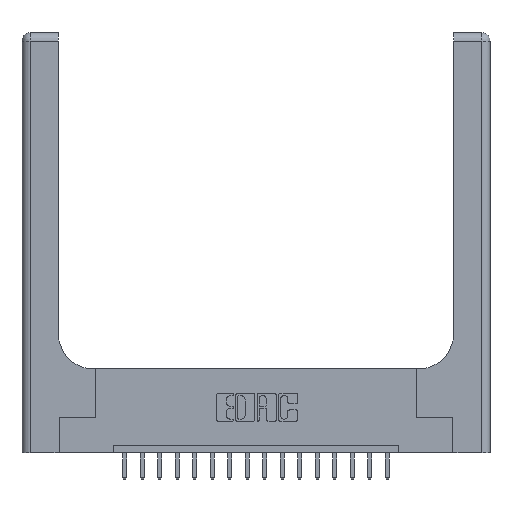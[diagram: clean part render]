
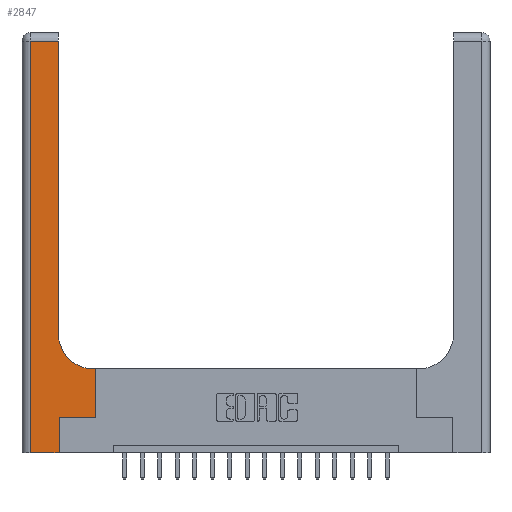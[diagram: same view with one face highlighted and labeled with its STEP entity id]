
A CAD part, top view. The second image highlights one B-rep face of the part: STEP entity #2847.
In plain terms, the highlighted planar face has unit normal (0, 0, 1).
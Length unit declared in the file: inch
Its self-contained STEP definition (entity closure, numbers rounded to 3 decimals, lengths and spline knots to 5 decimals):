
#92 = EDGE_CURVE ( 'NONE', #11981, #3421, #6889, .T. ) ;
#322 = EDGE_LOOP ( 'NONE', ( #5692, #11953, #2452, #6308, #9008, #10097, #18201, #10493, #4284 ) ) ;
#1026 = VERTEX_POINT ( 'NONE', #11431 ) ;
#1510 = DIRECTION ( 'NONE',  ( -1., 0., 0. ) ) ;
#1514 = DIRECTION ( 'NONE',  ( 0., -1., 0. ) ) ;
#1616 = CARTESIAN_POINT ( 'NONE',  ( 0.265, 0., 0.37 ) ) ;
#1628 = VECTOR ( 'NONE', #1514, 39.37008 ) ;
#1690 = CARTESIAN_POINT ( 'NONE',  ( 0., 0., 0.37 ) ) ;
#1723 = LINE ( 'NONE', #10750, #18697 ) ;
#1768 = EDGE_CURVE ( 'NONE', #16068, #11981, #5898, .T. ) ;
#2219 = AXIS2_PLACEMENT_3D ( 'NONE', #16606, #16136, #1510 ) ;
#2291 = VECTOR ( 'NONE', #14707, 39.37008 ) ;
#2452 = ORIENTED_EDGE ( 'NONE', *, *, #1768, .T. ) ;
#2787 = EDGE_CURVE ( 'NONE', #1026, #17145, #7936, .T. ) ;
#2847 = ADVANCED_FACE ( 'NONE', ( #5882 ), #9473, .F. ) ;
#3150 = CARTESIAN_POINT ( 'NONE',  ( 0.06, 2.94, 0.37 ) ) ;
#3396 = CARTESIAN_POINT ( 'NONE',  ( 0.06, 0., 0.37 ) ) ;
#3421 = VERTEX_POINT ( 'NONE', #1616 ) ;
#3450 = DIRECTION ( 'NONE',  ( -1., 0., 0. ) ) ;
#4181 = DIRECTION ( 'NONE',  ( 0., 1., 0. ) ) ;
#4243 = CARTESIAN_POINT ( 'NONE',  ( 0.26, 3., 0.37 ) ) ;
#4284 = ORIENTED_EDGE ( 'NONE', *, *, #16652, .T. ) ;
#4344 = CARTESIAN_POINT ( 'NONE',  ( 0.51, 0.85, 0.37 ) ) ;
#4393 = CARTESIAN_POINT ( 'NONE',  ( 0.26, 0.85, 0.37 ) ) ;
#4612 = DIRECTION ( 'NONE',  ( 1., 0., 0. ) ) ;
#4707 = LINE ( 'NONE', #17828, #12380 ) ;
#5012 = EDGE_CURVE ( 'NONE', #15742, #16068, #4707, .T. ) ;
#5066 = CARTESIAN_POINT ( 'NONE',  ( 0.26, 0.6, 0.37 ) ) ;
#5549 = VERTEX_POINT ( 'NONE', #12765 ) ;
#5692 = ORIENTED_EDGE ( 'NONE', *, *, #11798, .T. ) ;
#5882 = FACE_OUTER_BOUND ( 'NONE', #322, .T. ) ;
#5898 = LINE ( 'NONE', #17225, #1628 ) ;
#6308 = ORIENTED_EDGE ( 'NONE', *, *, #92, .T. ) ;
#6889 = LINE ( 'NONE', #1690, #17282 ) ;
#7333 = DIRECTION ( 'NONE',  ( 0., 0., -1. ) ) ;
#7592 = LINE ( 'NONE', #4243, #16417 ) ;
#7936 = LINE ( 'NONE', #10227, #2291 ) ;
#9008 = ORIENTED_EDGE ( 'NONE', *, *, #11992, .T. ) ;
#9453 = LINE ( 'NONE', #16576, #17805 ) ;
#9466 = DIRECTION ( 'NONE',  ( -1., 0., 0. ) ) ;
#9473 = PLANE ( 'NONE',  #2219 ) ;
#10071 = DIRECTION ( 'NONE',  ( 1., 0., 0. ) ) ;
#10097 = ORIENTED_EDGE ( 'NONE', *, *, #2787, .T. ) ;
#10227 = CARTESIAN_POINT ( 'NONE',  ( 0.265, 0.25, 0.37 ) ) ;
#10493 = ORIENTED_EDGE ( 'NONE', *, *, #15002, .T. ) ;
#10563 = DIRECTION ( 'NONE',  ( 0., 1., 0. ) ) ;
#10750 = CARTESIAN_POINT ( 'NONE',  ( 0.265, 0., 0.37 ) ) ;
#10831 = AXIS2_PLACEMENT_3D ( 'NONE', #4344, #7333, #10071 ) ;
#11431 = CARTESIAN_POINT ( 'NONE',  ( 0.265, 0.25, 0.37 ) ) ;
#11464 = VERTEX_POINT ( 'NONE', #4393 ) ;
#11509 = DIRECTION ( 'NONE',  ( 0., 1., 0. ) ) ;
#11798 = EDGE_CURVE ( 'NONE', #11464, #15742, #7592, .T. ) ;
#11953 = ORIENTED_EDGE ( 'NONE', *, *, #5012, .T. ) ;
#11981 = VERTEX_POINT ( 'NONE', #3396 ) ;
#11992 = EDGE_CURVE ( 'NONE', #3421, #1026, #1723, .T. ) ;
#12380 = VECTOR ( 'NONE', #3450, 39.37008 ) ;
#12381 = CARTESIAN_POINT ( 'NONE',  ( 0.51, 0.6, 0.37 ) ) ;
#12389 = VERTEX_POINT ( 'NONE', #12381 ) ;
#12765 = CARTESIAN_POINT ( 'NONE',  ( 0.528, 0.6, 0.37 ) ) ;
#13876 = CARTESIAN_POINT ( 'NONE',  ( 0.26, 2.94, 0.37 ) ) ;
#14017 = CIRCLE ( 'NONE', #10831, 0.25 ) ;
#14165 = CARTESIAN_POINT ( 'NONE',  ( 0.528, 0.25, 0.37 ) ) ;
#14707 = DIRECTION ( 'NONE',  ( 1., 0., 0. ) ) ;
#15002 = EDGE_CURVE ( 'NONE', #5549, #12389, #15394, .T. ) ;
#15394 = LINE ( 'NONE', #5066, #15618 ) ;
#15618 = VECTOR ( 'NONE', #9466, 39.37008 ) ;
#15742 = VERTEX_POINT ( 'NONE', #13876 ) ;
#16068 = VERTEX_POINT ( 'NONE', #3150 ) ;
#16136 = DIRECTION ( 'NONE',  ( 0., 0., -1. ) ) ;
#16417 = VECTOR ( 'NONE', #4181, 39.37008 ) ;
#16576 = CARTESIAN_POINT ( 'NONE',  ( 0.528, 0.25, 0.37 ) ) ;
#16606 = CARTESIAN_POINT ( 'NONE',  ( 0., 3., 0.37 ) ) ;
#16652 = EDGE_CURVE ( 'NONE', #12389, #11464, #14017, .T. ) ;
#17145 = VERTEX_POINT ( 'NONE', #14165 ) ;
#17225 = CARTESIAN_POINT ( 'NONE',  ( 0.06, 3., 0.37 ) ) ;
#17282 = VECTOR ( 'NONE', #4612, 39.37008 ) ;
#17730 = EDGE_CURVE ( 'NONE', #17145, #5549, #9453, .T. ) ;
#17805 = VECTOR ( 'NONE', #11509, 39.37008 ) ;
#17828 = CARTESIAN_POINT ( 'NONE',  ( 0., 2.94, 0.37 ) ) ;
#18201 = ORIENTED_EDGE ( 'NONE', *, *, #17730, .T. ) ;
#18697 = VECTOR ( 'NONE', #10563, 39.37008 ) ;
